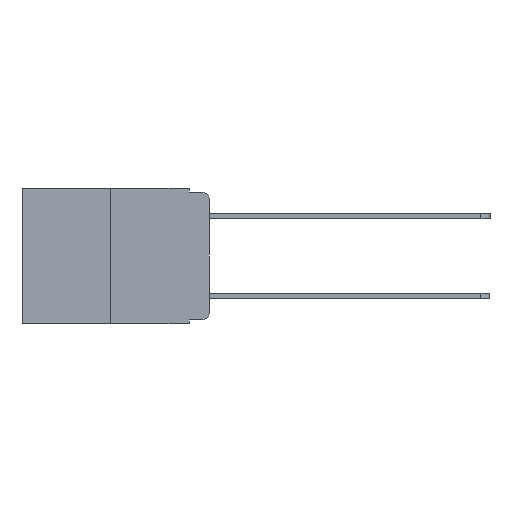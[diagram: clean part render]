
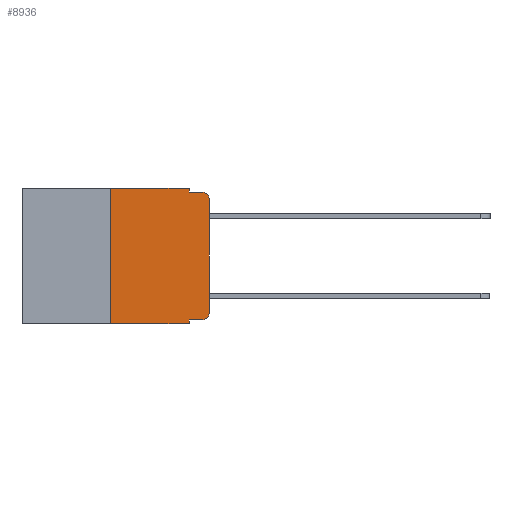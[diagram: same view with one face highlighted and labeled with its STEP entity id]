
A CAD part, left-side view. The second image highlights one B-rep face of the part: STEP entity #8936.
In plain terms, the highlighted planar face has unit normal (-1, 0, 0).
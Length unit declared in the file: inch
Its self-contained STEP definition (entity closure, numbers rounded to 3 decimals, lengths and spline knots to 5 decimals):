
#68 = VERTEX_POINT ( 'NONE', #10799 ) ;
#451 = CARTESIAN_POINT ( 'NONE',  ( 0., 0.051, -0.01 ) ) ;
#477 = CARTESIAN_POINT ( 'NONE',  ( 0., 0.25, -0.343 ) ) ;
#675 = PLANE ( 'NONE',  #4627 ) ;
#732 = VECTOR ( 'NONE', #5418, 39.37008 ) ;
#952 = VECTOR ( 'NONE', #7813, 39.37008 ) ;
#980 = DIRECTION ( 'NONE',  ( 0., 0., 1. ) ) ;
#1651 = CARTESIAN_POINT ( 'NONE',  ( 0., 0.02, -0.313 ) ) ;
#1848 = DIRECTION ( 'NONE',  ( 0., 0., -1. ) ) ;
#2001 = CARTESIAN_POINT ( 'NONE',  ( 0., 0.051, 0. ) ) ;
#2778 = EDGE_CURVE ( 'NONE', #5925, #9658, #6914, .T. ) ;
#2834 = VECTOR ( 'NONE', #8344, 39.37008 ) ;
#2889 = CARTESIAN_POINT ( 'NONE',  ( 0., 0.473, 0. ) ) ;
#2909 = CARTESIAN_POINT ( 'NONE',  ( 0., 0.473, -0.343 ) ) ;
#3287 = EDGE_CURVE ( 'NONE', #9658, #7026, #9540, .T. ) ;
#3630 = CARTESIAN_POINT ( 'NONE',  ( 0., 0.25, 0. ) ) ;
#3871 = VECTOR ( 'NONE', #9536, 39.37008 ) ;
#4461 = DIRECTION ( 'NONE',  ( 0., 0., -1. ) ) ;
#4627 = AXIS2_PLACEMENT_3D ( 'NONE', #2889, #7794, #1848 ) ;
#4942 = CARTESIAN_POINT ( 'NONE',  ( 0., 0.051, 0. ) ) ;
#5191 = CARTESIAN_POINT ( 'NONE',  ( 0., 0.02, -0.03 ) ) ;
#5332 = VECTOR ( 'NONE', #10265, 39.37008 ) ;
#5418 = DIRECTION ( 'NONE',  ( 0., -1., 0. ) ) ;
#5551 = CARTESIAN_POINT ( 'NONE',  ( 0., 0.051, -0.333 ) ) ;
#5619 = LINE ( 'NONE', #3630, #2834 ) ;
#5673 = VERTEX_POINT ( 'NONE', #6384 ) ;
#5773 = LINE ( 'NONE', #7149, #7874 ) ;
#5925 = VERTEX_POINT ( 'NONE', #8091 ) ;
#6037 = FACE_OUTER_BOUND ( 'NONE', #7533, .T. ) ;
#6064 = EDGE_CURVE ( 'NONE', #10950, #68, #8860, .T. ) ;
#6124 = DIRECTION ( 'NONE',  ( 0., 0., -1. ) ) ;
#6235 = CARTESIAN_POINT ( 'NONE',  ( 0., 0.051, -0.343 ) ) ;
#6306 = CARTESIAN_POINT ( 'NONE',  ( 0., 0., -0.313 ) ) ;
#6384 = CARTESIAN_POINT ( 'NONE',  ( 0., 0., -0.03 ) ) ;
#6406 = ORIENTED_EDGE ( 'NONE', *, *, #12361, .F. ) ;
#6633 = CIRCLE ( 'NONE', #10724, 0.02 ) ;
#6885 = LINE ( 'NONE', #10026, #7164 ) ;
#6902 = VECTOR ( 'NONE', #8487, 39.37008 ) ;
#6914 = LINE ( 'NONE', #5551, #732 ) ;
#7026 = VERTEX_POINT ( 'NONE', #6306 ) ;
#7149 = CARTESIAN_POINT ( 'NONE',  ( 0., 0., 0. ) ) ;
#7164 = VECTOR ( 'NONE', #10893, 39.37008 ) ;
#7533 = EDGE_LOOP ( 'NONE', ( #11498, #11440, #6406, #10046, #9727, #9743, #9776, #10207, #9765, #11275 ) ) ;
#7639 = CARTESIAN_POINT ( 'NONE',  ( 0., 0.051, 0. ) ) ;
#7794 = DIRECTION ( 'NONE',  ( 1., 0., 0. ) ) ;
#7813 = DIRECTION ( 'NONE',  ( 0., 0., -1. ) ) ;
#7874 = VECTOR ( 'NONE', #980, 39.37008 ) ;
#8091 = CARTESIAN_POINT ( 'NONE',  ( 0., 0.051, -0.333 ) ) ;
#8344 = DIRECTION ( 'NONE',  ( 0., 0., 1. ) ) ;
#8449 = EDGE_CURVE ( 'NONE', #8764, #9127, #8531, .T. ) ;
#8487 = DIRECTION ( 'NONE',  ( 0., -1., 0. ) ) ;
#8531 = LINE ( 'NONE', #2909, #3871 ) ;
#8764 = VERTEX_POINT ( 'NONE', #477 ) ;
#8860 = LINE ( 'NONE', #7639, #952 ) ;
#8936 = ADVANCED_FACE ( 'NONE', ( #6037 ), #675, .F. ) ;
#9116 = VERTEX_POINT ( 'NONE', #9702 ) ;
#9127 = VERTEX_POINT ( 'NONE', #6235 ) ;
#9448 = EDGE_CURVE ( 'NONE', #9116, #10950, #6885, .T. ) ;
#9493 = LINE ( 'NONE', #451, #6902 ) ;
#9536 = DIRECTION ( 'NONE',  ( 0., -1., 0. ) ) ;
#9540 = CIRCLE ( 'NONE', #11851, 0.02 ) ;
#9658 = VERTEX_POINT ( 'NONE', #11913 ) ;
#9702 = CARTESIAN_POINT ( 'NONE',  ( 0., 0.25, 0. ) ) ;
#9727 = ORIENTED_EDGE ( 'NONE', *, *, #9448, .F. ) ;
#9743 = ORIENTED_EDGE ( 'NONE', *, *, #11304, .F. ) ;
#9765 = ORIENTED_EDGE ( 'NONE', *, *, #2778, .T. ) ;
#9776 = ORIENTED_EDGE ( 'NONE', *, *, #8449, .T. ) ;
#10026 = CARTESIAN_POINT ( 'NONE',  ( 0., 0.473, 0. ) ) ;
#10046 = ORIENTED_EDGE ( 'NONE', *, *, #6064, .F. ) ;
#10207 = ORIENTED_EDGE ( 'NONE', *, *, #11449, .F. ) ;
#10265 = DIRECTION ( 'NONE',  ( 0., 0., -1. ) ) ;
#10724 = AXIS2_PLACEMENT_3D ( 'NONE', #5191, #11336, #6124 ) ;
#10799 = CARTESIAN_POINT ( 'NONE',  ( 0., 0.051, -0.01 ) ) ;
#10891 = EDGE_CURVE ( 'NONE', #5673, #12398, #6633, .T. ) ;
#10893 = DIRECTION ( 'NONE',  ( 0., -1., 0. ) ) ;
#10950 = VERTEX_POINT ( 'NONE', #2001 ) ;
#11048 = EDGE_CURVE ( 'NONE', #7026, #5673, #5773, .T. ) ;
#11275 = ORIENTED_EDGE ( 'NONE', *, *, #3287, .T. ) ;
#11304 = EDGE_CURVE ( 'NONE', #8764, #9116, #5619, .T. ) ;
#11336 = DIRECTION ( 'NONE',  ( -1., 0., 0. ) ) ;
#11440 = ORIENTED_EDGE ( 'NONE', *, *, #10891, .T. ) ;
#11449 = EDGE_CURVE ( 'NONE', #5925, #9127, #11758, .T. ) ;
#11498 = ORIENTED_EDGE ( 'NONE', *, *, #11048, .T. ) ;
#11758 = LINE ( 'NONE', #4942, #5332 ) ;
#11851 = AXIS2_PLACEMENT_3D ( 'NONE', #1651, #12320, #4461 ) ;
#11913 = CARTESIAN_POINT ( 'NONE',  ( 0., 0.02, -0.333 ) ) ;
#11962 = CARTESIAN_POINT ( 'NONE',  ( 0., 0.02, -0.01 ) ) ;
#12320 = DIRECTION ( 'NONE',  ( -1., 0., 0. ) ) ;
#12361 = EDGE_CURVE ( 'NONE', #68, #12398, #9493, .T. ) ;
#12398 = VERTEX_POINT ( 'NONE', #11962 ) ;
